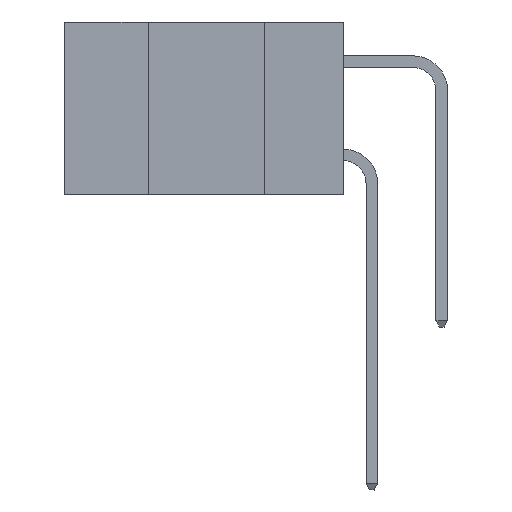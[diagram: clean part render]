
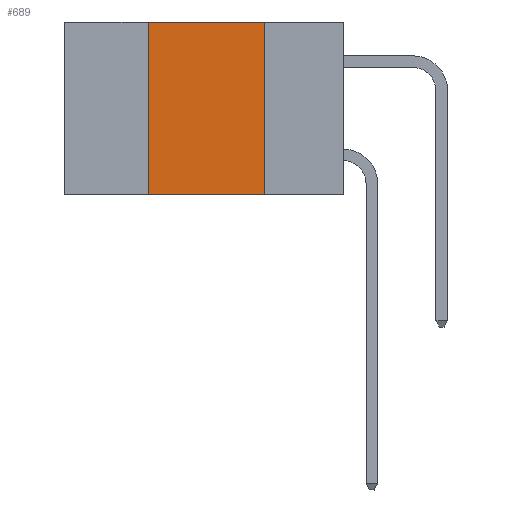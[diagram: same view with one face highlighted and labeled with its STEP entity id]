
A CAD part, left-side view. The second image highlights one B-rep face of the part: STEP entity #689.
In plain terms, the highlighted planar face has unit normal (-1, 0, 0).
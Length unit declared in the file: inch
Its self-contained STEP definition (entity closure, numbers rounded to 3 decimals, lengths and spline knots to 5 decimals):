
#303 = ORIENTED_EDGE ( 'NONE', *, *, #15825, .F. ) ;
#689 = ADVANCED_FACE ( 'NONE', ( #11676 ), #19123, .F. ) ;
#1552 = EDGE_CURVE ( 'NONE', #5089, #8617, #5838, .T. ) ;
#2568 = VECTOR ( 'NONE', #12293, 39.37008 ) ;
#3187 = ORIENTED_EDGE ( 'NONE', *, *, #12240, .F. ) ;
#3898 = CARTESIAN_POINT ( 'NONE',  ( 0., 0.42, 0. ) ) ;
#4167 = VECTOR ( 'NONE', #6834, 39.37008 ) ;
#5089 = VERTEX_POINT ( 'NONE', #3898 ) ;
#5159 = VECTOR ( 'NONE', #6753, 39.37008 ) ;
#5390 = CARTESIAN_POINT ( 'NONE',  ( 0., 0.42, -0.37 ) ) ;
#5472 = DIRECTION ( 'NONE',  ( 0., -1., 0. ) ) ;
#5838 = LINE ( 'NONE', #20618, #19693 ) ;
#6043 = ORIENTED_EDGE ( 'NONE', *, *, #1552, .F. ) ;
#6675 = CARTESIAN_POINT ( 'NONE',  ( 0., 0.17, -0.37 ) ) ;
#6753 = DIRECTION ( 'NONE',  ( 0., 0., -1. ) ) ;
#6760 = VERTEX_POINT ( 'NONE', #5390 ) ;
#6834 = DIRECTION ( 'NONE',  ( 0., -1., 0. ) ) ;
#7056 = EDGE_LOOP ( 'NONE', ( #3187, #6043, #303, #15218 ) ) ;
#7470 = DIRECTION ( 'NONE',  ( 0., 0., -1. ) ) ;
#8617 = VERTEX_POINT ( 'NONE', #9282 ) ;
#9282 = CARTESIAN_POINT ( 'NONE',  ( 0., 0.17, 0. ) ) ;
#9447 = DIRECTION ( 'NONE',  ( 1., 0., 0. ) ) ;
#9797 = VERTEX_POINT ( 'NONE', #6675 ) ;
#10611 = CARTESIAN_POINT ( 'NONE',  ( 0., 0.17, -0.37 ) ) ;
#11676 = FACE_OUTER_BOUND ( 'NONE', #7056, .T. ) ;
#12240 = EDGE_CURVE ( 'NONE', #8617, #9797, #14461, .T. ) ;
#12293 = DIRECTION ( 'NONE',  ( 0., 0., 1. ) ) ;
#14127 = AXIS2_PLACEMENT_3D ( 'NONE', #23083, #9447, #7470 ) ;
#14271 = CARTESIAN_POINT ( 'NONE',  ( 0., 0.42, -0.37 ) ) ;
#14461 = LINE ( 'NONE', #10611, #5159 ) ;
#14645 = LINE ( 'NONE', #23848, #4167 ) ;
#15218 = ORIENTED_EDGE ( 'NONE', *, *, #23849, .T. ) ;
#15825 = EDGE_CURVE ( 'NONE', #6760, #5089, #16012, .T. ) ;
#16012 = LINE ( 'NONE', #14271, #2568 ) ;
#19123 = PLANE ( 'NONE',  #14127 ) ;
#19693 = VECTOR ( 'NONE', #5472, 39.37008 ) ;
#20618 = CARTESIAN_POINT ( 'NONE',  ( 0., 0.6, 0. ) ) ;
#23083 = CARTESIAN_POINT ( 'NONE',  ( 0., 0.6, 0. ) ) ;
#23848 = CARTESIAN_POINT ( 'NONE',  ( 0., 0.6, -0.37 ) ) ;
#23849 = EDGE_CURVE ( 'NONE', #6760, #9797, #14645, .T. ) ;
